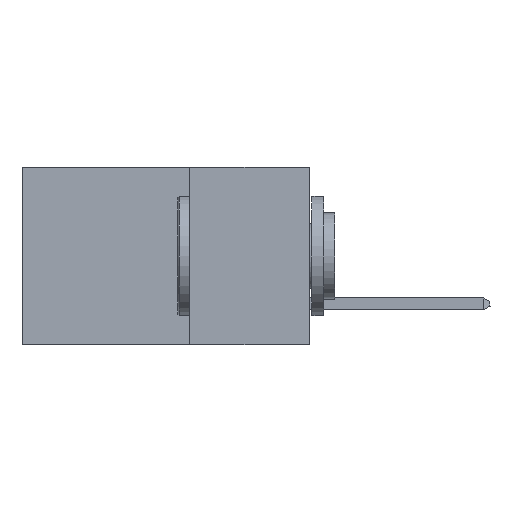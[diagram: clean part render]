
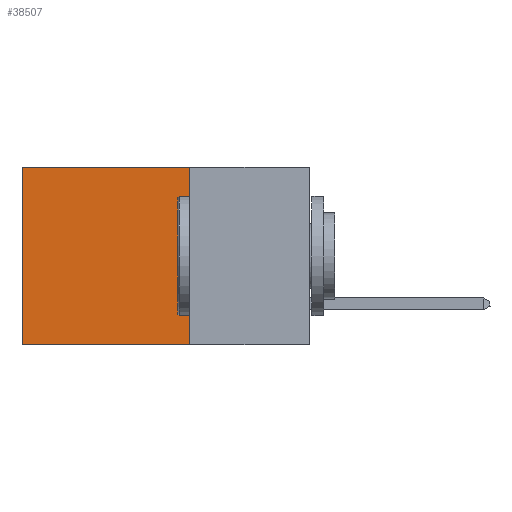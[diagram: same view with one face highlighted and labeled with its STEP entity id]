
A CAD part, left-side view. The second image highlights one B-rep face of the part: STEP entity #38507.
In plain terms, the highlighted planar face has unit normal (-1, 0, 0).
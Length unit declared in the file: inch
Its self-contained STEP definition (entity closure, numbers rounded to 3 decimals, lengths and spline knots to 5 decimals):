
#237 = VECTOR ( 'NONE', #45128, 39.37008 ) ;
#868 = VERTEX_POINT ( 'NONE', #43022 ) ;
#2068 = VECTOR ( 'NONE', #8400, 39.37008 ) ;
#4611 = CARTESIAN_POINT ( 'NONE',  ( 0.2875, 0.25, -0.37 ) ) ;
#6006 = LINE ( 'NONE', #6141, #45107 ) ;
#6141 = CARTESIAN_POINT ( 'NONE',  ( 0.2875, 0.6, 0. ) ) ;
#6614 = CARTESIAN_POINT ( 'NONE',  ( 0.2875, 0.6, 0. ) ) ;
#6911 = VERTEX_POINT ( 'NONE', #37563 ) ;
#8150 = ORIENTED_EDGE ( 'NONE', *, *, #24951, .F. ) ;
#8400 = DIRECTION ( 'NONE',  ( 0., 1., 0. ) ) ;
#10053 = EDGE_CURVE ( 'NONE', #28616, #868, #21618, .T. ) ;
#10526 = DIRECTION ( 'NONE',  ( 0., 0., -1. ) ) ;
#11863 = AXIS2_PLACEMENT_3D ( 'NONE', #33554, #44854, #10526 ) ;
#12388 = VECTOR ( 'NONE', #46703, 39.37008 ) ;
#13766 = DIRECTION ( 'NONE',  ( 0., 0., -1. ) ) ;
#20094 = FACE_OUTER_BOUND ( 'NONE', #45683, .T. ) ;
#21250 = EDGE_CURVE ( 'NONE', #6911, #22389, #36110, .T. ) ;
#21532 = PLANE ( 'NONE',  #11863 ) ;
#21618 = LINE ( 'NONE', #4611, #2068 ) ;
#22389 = VERTEX_POINT ( 'NONE', #6614 ) ;
#24063 = ORIENTED_EDGE ( 'NONE', *, *, #36405, .T. ) ;
#24951 = EDGE_CURVE ( 'NONE', #6911, #28616, #41713, .T. ) ;
#27633 = CARTESIAN_POINT ( 'NONE',  ( 0.2875, 0.25, 0. ) ) ;
#28616 = VERTEX_POINT ( 'NONE', #32402 ) ;
#30797 = ORIENTED_EDGE ( 'NONE', *, *, #21250, .T. ) ;
#32402 = CARTESIAN_POINT ( 'NONE',  ( 0.2875, 0.25, -0.37 ) ) ;
#33554 = CARTESIAN_POINT ( 'NONE',  ( 0.2875, 0.25, 0. ) ) ;
#36110 = LINE ( 'NONE', #27633, #12388 ) ;
#36405 = EDGE_CURVE ( 'NONE', #22389, #868, #6006, .T. ) ;
#37563 = CARTESIAN_POINT ( 'NONE',  ( 0.2875, 0.25, 0. ) ) ;
#38507 = ADVANCED_FACE ( 'NONE', ( #20094 ), #21532, .F. ) ;
#41713 = LINE ( 'NONE', #45294, #237 ) ;
#43022 = CARTESIAN_POINT ( 'NONE',  ( 0.2875, 0.6, -0.37 ) ) ;
#44854 = DIRECTION ( 'NONE',  ( 1., 0., 0. ) ) ;
#45107 = VECTOR ( 'NONE', #13766, 39.37008 ) ;
#45128 = DIRECTION ( 'NONE',  ( 0., 0., -1. ) ) ;
#45294 = CARTESIAN_POINT ( 'NONE',  ( 0.2875, 0.25, 0. ) ) ;
#45683 = EDGE_LOOP ( 'NONE', ( #24063, #47174, #8150, #30797 ) ) ;
#46703 = DIRECTION ( 'NONE',  ( 0., 1., 0. ) ) ;
#47174 = ORIENTED_EDGE ( 'NONE', *, *, #10053, .F. ) ;
